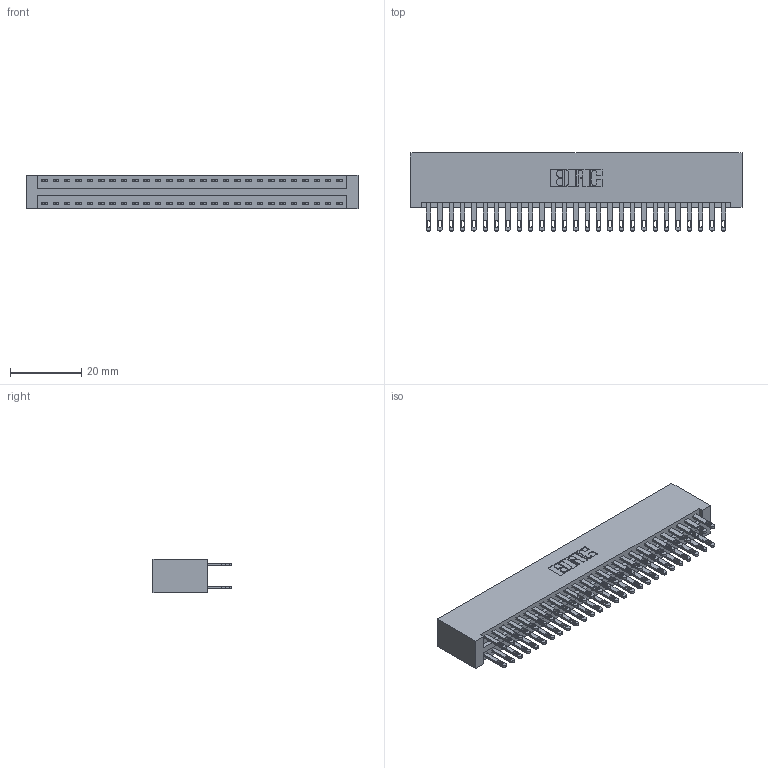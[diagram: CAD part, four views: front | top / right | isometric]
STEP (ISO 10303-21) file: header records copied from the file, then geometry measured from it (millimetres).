
FILE_DESCRIPTION (( 'STEP AP203' ), '1' );
FILE_NAME ('896-054-500-201.STEP', '2021-07-27T23:50:59', ( '' ), ( '' ), 'SwSTEP 2.0', 'SolidWorks 2020', '' );
FILE_SCHEMA (( 'CONFIG_CONTROL_DESIGN' ));
Length unit declared in the file: inch
Products named in the file (3): 846 Part_No Mounting Lugs; 896-054-500-201; 345-292-001_345-293-100
Assembly tree (55 placements, depth 2):
  896-054-500-201
    846 Part_No Mounting Lugs
    345-292-001_345-293-100  x54
Bounding box: 92.96 x 21.84 x 9.4 mm (x, y, z)
Volume: 9686.9 mm3; surface area: 13808 mm2
Topology: 55 solids, 55 shells, 2706 faces, 8243 edges, 5494 vertices
Faces by surface type: plane 1638, cylinder 1068
Entity records: 19293 total; most frequent: CARTESIAN_POINT 3196, ORIENTED_EDGE 3130, DIRECTION 2865, EDGE_CURVE 1565, LINE 1329, VECTOR 1329, VERTEX_POINT 1042, AXIS2_PLACEMENT_3D 768
